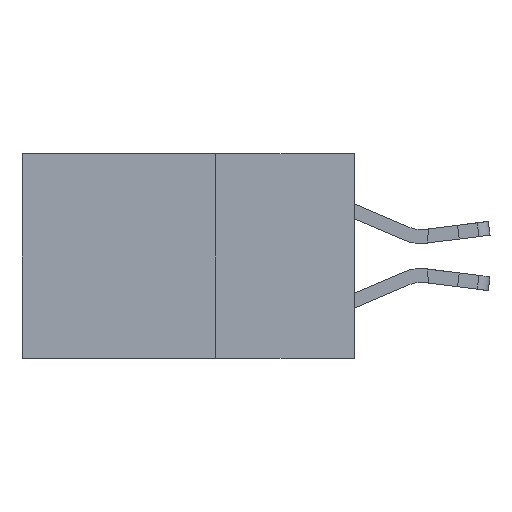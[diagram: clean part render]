
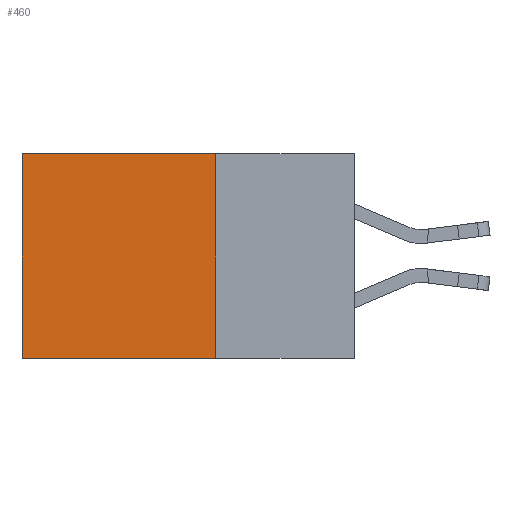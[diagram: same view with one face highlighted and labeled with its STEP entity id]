
A CAD part, left-side view. The second image highlights one B-rep face of the part: STEP entity #460.
In plain terms, the highlighted planar face has unit normal (-1, 0, 0).
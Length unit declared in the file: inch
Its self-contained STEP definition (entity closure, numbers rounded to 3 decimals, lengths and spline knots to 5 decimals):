
#60 = EDGE_CURVE ( 'NONE', #2180, #7355, #7587, .T. ) ;
#460 = ADVANCED_FACE ( 'NONE', ( #4434 ), #2558, .F. ) ;
#1688 = VECTOR ( 'NONE', #10437, 39.37008 ) ;
#1813 = DIRECTION ( 'NONE',  ( 1., 0., 0. ) ) ;
#2180 = VERTEX_POINT ( 'NONE', #4425 ) ;
#2558 = PLANE ( 'NONE',  #6661 ) ;
#3289 = EDGE_CURVE ( 'NONE', #2180, #10379, #6573, .T. ) ;
#4215 = DIRECTION ( 'NONE',  ( 0., 1., 0. ) ) ;
#4425 = CARTESIAN_POINT ( 'NONE',  ( 0.2615, 0.25, 0. ) ) ;
#4434 = FACE_OUTER_BOUND ( 'NONE', #9518, .T. ) ;
#4757 = CARTESIAN_POINT ( 'NONE',  ( 0.2615, 0.25, -0.37 ) ) ;
#4934 = VERTEX_POINT ( 'NONE', #8449 ) ;
#4946 = CARTESIAN_POINT ( 'NONE',  ( 0.2615, 0.25, -0.37 ) ) ;
#5089 = EDGE_CURVE ( 'NONE', #7355, #4934, #9587, .T. ) ;
#5470 = DIRECTION ( 'NONE',  ( 0., 0., -1. ) ) ;
#5601 = DIRECTION ( 'NONE',  ( 0., 0., -1. ) ) ;
#5720 = DIRECTION ( 'NONE',  ( 0., 1., 0. ) ) ;
#6009 = ORIENTED_EDGE ( 'NONE', *, *, #6374, .F. ) ;
#6374 = EDGE_CURVE ( 'NONE', #10379, #4934, #10558, .T. ) ;
#6573 = LINE ( 'NONE', #4757, #9840 ) ;
#6661 = AXIS2_PLACEMENT_3D ( 'NONE', #11746, #1813, #5470 ) ;
#7316 = CARTESIAN_POINT ( 'NONE',  ( 0.2615, 0.25, -0.37 ) ) ;
#7355 = VERTEX_POINT ( 'NONE', #10765 ) ;
#7587 = LINE ( 'NONE', #9503, #10975 ) ;
#7842 = ORIENTED_EDGE ( 'NONE', *, *, #60, .T. ) ;
#7847 = CARTESIAN_POINT ( 'NONE',  ( 0.2615, 0.6, -0.37 ) ) ;
#7920 = ORIENTED_EDGE ( 'NONE', *, *, #3289, .F. ) ;
#8449 = CARTESIAN_POINT ( 'NONE',  ( 0.2615, 0.6, -0.37 ) ) ;
#8858 = ORIENTED_EDGE ( 'NONE', *, *, #5089, .T. ) ;
#9503 = CARTESIAN_POINT ( 'NONE',  ( 0.2615, 0.25, 0. ) ) ;
#9518 = EDGE_LOOP ( 'NONE', ( #8858, #6009, #7920, #7842 ) ) ;
#9587 = LINE ( 'NONE', #7847, #1688 ) ;
#9840 = VECTOR ( 'NONE', #5601, 39.37008 ) ;
#10379 = VERTEX_POINT ( 'NONE', #7316 ) ;
#10437 = DIRECTION ( 'NONE',  ( 0., 0., -1. ) ) ;
#10558 = LINE ( 'NONE', #4946, #11172 ) ;
#10765 = CARTESIAN_POINT ( 'NONE',  ( 0.2615, 0.6, 0. ) ) ;
#10975 = VECTOR ( 'NONE', #5720, 39.37008 ) ;
#11172 = VECTOR ( 'NONE', #4215, 39.37008 ) ;
#11746 = CARTESIAN_POINT ( 'NONE',  ( 0.2615, 0.25, -0.37 ) ) ;
